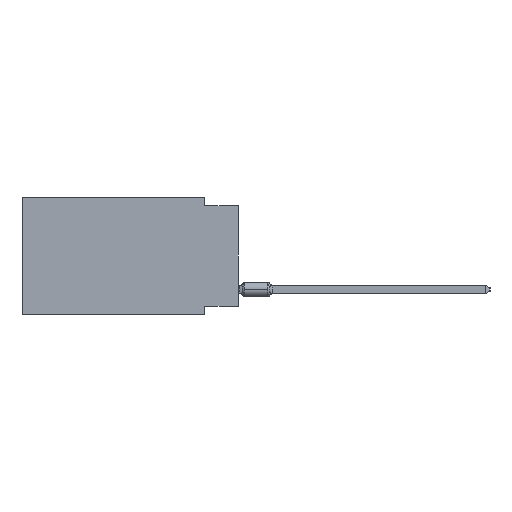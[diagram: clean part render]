
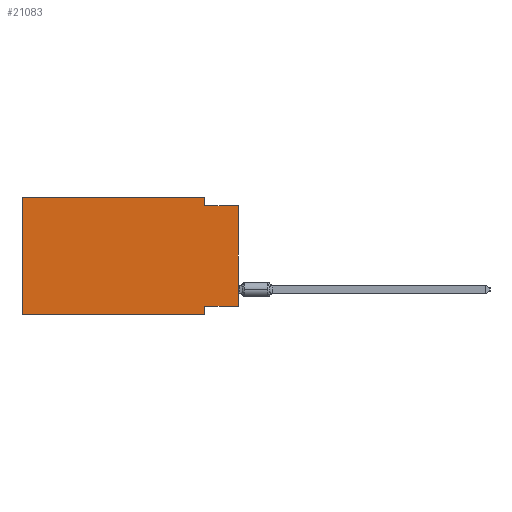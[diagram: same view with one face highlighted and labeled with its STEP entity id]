
A CAD part, left-side view. The second image highlights one B-rep face of the part: STEP entity #21083.
In plain terms, the highlighted planar face has unit normal (-1, 0, 0).
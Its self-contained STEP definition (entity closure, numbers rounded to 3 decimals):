
#174 = VECTOR ( 'NONE', #89996, 1000. ) ;
#402 = CARTESIAN_POINT ( 'NONE',  ( 0., 16.383, 0. ) ) ;
#1270 = VERTEX_POINT ( 'NONE', #3750 ) ;
#2661 = VECTOR ( 'NONE', #36247, 1000. ) ;
#3750 = CARTESIAN_POINT ( 'NONE',  ( 0., 2.54, -0.635 ) ) ;
#4871 = EDGE_CURVE ( 'NONE', #45771, #44706, #9190, .T. ) ;
#5490 = LINE ( 'NONE', #87695, #55236 ) ;
#6917 = CARTESIAN_POINT ( 'NONE',  ( 0., 2.54, 0. ) ) ;
#9190 = LINE ( 'NONE', #25532, #66159 ) ;
#10153 = ORIENTED_EDGE ( 'NONE', *, *, #40200, .F. ) ;
#11670 = CARTESIAN_POINT ( 'NONE',  ( 0., 16.383, -8.89 ) ) ;
#11802 = AXIS2_PLACEMENT_3D ( 'NONE', #73264, #58367, #87715 ) ;
#13615 = LINE ( 'NONE', #21303, #64237 ) ;
#14120 = LINE ( 'NONE', #6917, #2661 ) ;
#14409 = EDGE_CURVE ( 'NONE', #39333, #49296, #60662, .T. ) ;
#17370 = CARTESIAN_POINT ( 'NONE',  ( 0., 0., 0. ) ) ;
#21083 = ADVANCED_FACE ( 'NONE', ( #67481 ), #29049, .F. ) ;
#21303 = CARTESIAN_POINT ( 'NONE',  ( 0., 2.54, -8.89 ) ) ;
#24302 = EDGE_CURVE ( 'NONE', #47809, #50624, #13615, .T. ) ;
#25531 = EDGE_LOOP ( 'NONE', ( #46083, #70471, #53072, #10153, #26533, #62189, #85645, #93864 ) ) ;
#25532 = CARTESIAN_POINT ( 'NONE',  ( 0., 16.383, 0. ) ) ;
#26533 = ORIENTED_EDGE ( 'NONE', *, *, #4871, .F. ) ;
#28437 = CARTESIAN_POINT ( 'NONE',  ( 0., 16.383, -8.89 ) ) ;
#28714 = VECTOR ( 'NONE', #35981, 1000. ) ;
#28909 = LINE ( 'NONE', #28437, #37498 ) ;
#29049 = PLANE ( 'NONE',  #11802 ) ;
#29967 = CARTESIAN_POINT ( 'NONE',  ( 0., 2.54, -8.89 ) ) ;
#32758 = DIRECTION ( 'NONE',  ( 0., 0., 1. ) ) ;
#35981 = DIRECTION ( 'NONE',  ( 0., -1., 0. ) ) ;
#36247 = DIRECTION ( 'NONE',  ( 0., 0., -1. ) ) ;
#37163 = CARTESIAN_POINT ( 'NONE',  ( 0., 0., -8.255 ) ) ;
#37498 = VECTOR ( 'NONE', #79865, 1000. ) ;
#37650 = VECTOR ( 'NONE', #82532, 1000. ) ;
#39333 = VERTEX_POINT ( 'NONE', #37163 ) ;
#40200 = EDGE_CURVE ( 'NONE', #44706, #48346, #78335, .T. ) ;
#44706 = VERTEX_POINT ( 'NONE', #402 ) ;
#45483 = LINE ( 'NONE', #59445, #37650 ) ;
#45771 = VERTEX_POINT ( 'NONE', #11670 ) ;
#46083 = ORIENTED_EDGE ( 'NONE', *, *, #14409, .T. ) ;
#47809 = VERTEX_POINT ( 'NONE', #86967 ) ;
#48346 = VERTEX_POINT ( 'NONE', #66629 ) ;
#48633 = EDGE_CURVE ( 'NONE', #45771, #50624, #28909, .T. ) ;
#49296 = VERTEX_POINT ( 'NONE', #60978 ) ;
#50624 = VERTEX_POINT ( 'NONE', #29967 ) ;
#53072 = ORIENTED_EDGE ( 'NONE', *, *, #53225, .F. ) ;
#53225 = EDGE_CURVE ( 'NONE', #48346, #1270, #14120, .T. ) ;
#55236 = VECTOR ( 'NONE', #73246, 1000. ) ;
#55988 = DIRECTION ( 'NONE',  ( 0., 0., -1. ) ) ;
#58367 = DIRECTION ( 'NONE',  ( 1., 0., 0. ) ) ;
#59445 = CARTESIAN_POINT ( 'NONE',  ( 0., 0., -0.635 ) ) ;
#60662 = LINE ( 'NONE', #17370, #174 ) ;
#60978 = CARTESIAN_POINT ( 'NONE',  ( 0., 0., -0.635 ) ) ;
#62189 = ORIENTED_EDGE ( 'NONE', *, *, #48633, .T. ) ;
#64237 = VECTOR ( 'NONE', #55988, 1000. ) ;
#66159 = VECTOR ( 'NONE', #32758, 1000. ) ;
#66629 = CARTESIAN_POINT ( 'NONE',  ( 0., 2.54, 0. ) ) ;
#67481 = FACE_OUTER_BOUND ( 'NONE', #25531, .T. ) ;
#68850 = EDGE_CURVE ( 'NONE', #1270, #49296, #45483, .T. ) ;
#70471 = ORIENTED_EDGE ( 'NONE', *, *, #68850, .F. ) ;
#73246 = DIRECTION ( 'NONE',  ( 0., 1., 0. ) ) ;
#73264 = CARTESIAN_POINT ( 'NONE',  ( 0., 16.383, 0. ) ) ;
#73378 = EDGE_CURVE ( 'NONE', #39333, #47809, #5490, .T. ) ;
#78335 = LINE ( 'NONE', #93707, #28714 ) ;
#79865 = DIRECTION ( 'NONE',  ( 0., -1., 0. ) ) ;
#82532 = DIRECTION ( 'NONE',  ( 0., -1., 0. ) ) ;
#85645 = ORIENTED_EDGE ( 'NONE', *, *, #24302, .F. ) ;
#86967 = CARTESIAN_POINT ( 'NONE',  ( 0., 2.54, -8.255 ) ) ;
#87695 = CARTESIAN_POINT ( 'NONE',  ( 0., 0., -8.255 ) ) ;
#87715 = DIRECTION ( 'NONE',  ( 0., 0., -1. ) ) ;
#89996 = DIRECTION ( 'NONE',  ( 0., 0., 1. ) ) ;
#93707 = CARTESIAN_POINT ( 'NONE',  ( 0., 16.383, 0. ) ) ;
#93864 = ORIENTED_EDGE ( 'NONE', *, *, #73378, .F. ) ;
